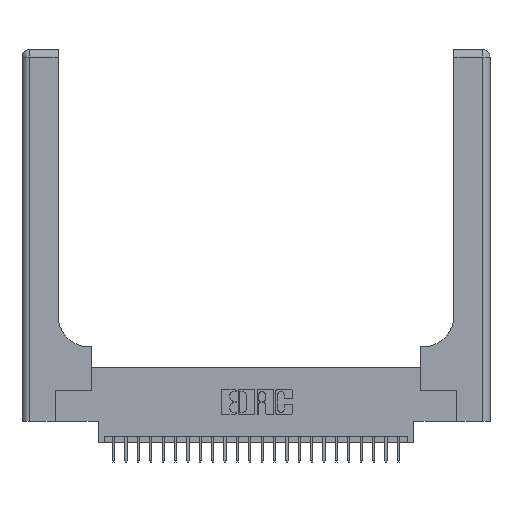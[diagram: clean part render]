
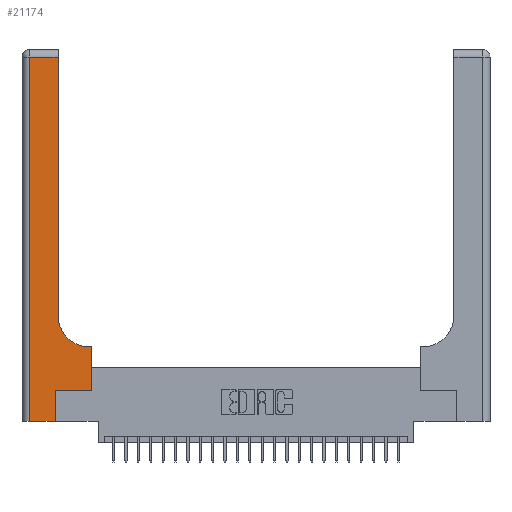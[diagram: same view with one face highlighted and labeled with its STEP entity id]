
A CAD part, top view. The second image highlights one B-rep face of the part: STEP entity #21174.
In plain terms, the highlighted planar face has unit normal (0, 0, 1).
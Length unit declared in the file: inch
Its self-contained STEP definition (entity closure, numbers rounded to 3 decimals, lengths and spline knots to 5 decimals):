
#319 = ORIENTED_EDGE ( 'NONE', *, *, #24677, .T. ) ;
#359 = EDGE_CURVE ( 'NONE', #11585, #13888, #10658, .T. ) ;
#406 = LINE ( 'NONE', #7875, #26483 ) ;
#523 = VECTOR ( 'NONE', #21432, 39.37008 ) ;
#627 = CARTESIAN_POINT ( 'NONE',  ( 0.269, 0.25, 0.37 ) ) ;
#949 = CARTESIAN_POINT ( 'NONE',  ( 0.5585, 0.25, 0.37 ) ) ;
#1217 = VERTEX_POINT ( 'NONE', #949 ) ;
#1274 = DIRECTION ( 'NONE',  ( -1., 0., 0. ) ) ;
#1945 = ORIENTED_EDGE ( 'NONE', *, *, #11618, .T. ) ;
#2642 = VERTEX_POINT ( 'NONE', #21640 ) ;
#3559 = VECTOR ( 'NONE', #11479, 39.37008 ) ;
#4810 = VECTOR ( 'NONE', #11477, 39.37008 ) ;
#5757 = VECTOR ( 'NONE', #14458, 39.37008 ) ;
#5876 = VECTOR ( 'NONE', #16796, 39.37008 ) ;
#6149 = LINE ( 'NONE', #627, #523 ) ;
#6441 = CARTESIAN_POINT ( 'NONE',  ( 0., 2.94, 0.37 ) ) ;
#6679 = CARTESIAN_POINT ( 'NONE',  ( 0.5415, 0.6, 0.37 ) ) ;
#7041 = EDGE_CURVE ( 'NONE', #7505, #15635, #25045, .T. ) ;
#7311 = AXIS2_PLACEMENT_3D ( 'NONE', #7810, #22193, #9916 ) ;
#7505 = VERTEX_POINT ( 'NONE', #21081 ) ;
#7810 = CARTESIAN_POINT ( 'NONE',  ( 0.5415, 0.85, 0.37 ) ) ;
#7875 = CARTESIAN_POINT ( 'NONE',  ( 0., 0., 0.37 ) ) ;
#8294 = AXIS2_PLACEMENT_3D ( 'NONE', #25908, #13824, #1274 ) ;
#8312 = VECTOR ( 'NONE', #22910, 39.37008 ) ;
#8372 = ORIENTED_EDGE ( 'NONE', *, *, #17217, .T. ) ;
#8820 = CARTESIAN_POINT ( 'NONE',  ( 0.2915, 2.94, 0.37 ) ) ;
#9391 = CARTESIAN_POINT ( 'NONE',  ( 0.5585, 0.25, 0.37 ) ) ;
#9601 = DIRECTION ( 'NONE',  ( 0., -1., 0. ) ) ;
#9610 = LINE ( 'NONE', #6441, #8312 ) ;
#9672 = EDGE_CURVE ( 'NONE', #2642, #1217, #6149, .T. ) ;
#9916 = DIRECTION ( 'NONE',  ( 1., 0., 0. ) ) ;
#10237 = VERTEX_POINT ( 'NONE', #8820 ) ;
#10658 = LINE ( 'NONE', #14487, #5757 ) ;
#11477 = DIRECTION ( 'NONE',  ( 0., 1., 0. ) ) ;
#11479 = DIRECTION ( 'NONE',  ( 0., 1., 0. ) ) ;
#11585 = VERTEX_POINT ( 'NONE', #22264 ) ;
#11618 = EDGE_CURVE ( 'NONE', #15635, #26148, #406, .T. ) ;
#11753 = PLANE ( 'NONE',  #8294 ) ;
#11860 = CARTESIAN_POINT ( 'NONE',  ( 0.269, 0., 0.37 ) ) ;
#12709 = ORIENTED_EDGE ( 'NONE', *, *, #359, .T. ) ;
#12786 = CIRCLE ( 'NONE', #7311, 0.25 ) ;
#13824 = DIRECTION ( 'NONE',  ( 0., 0., -1. ) ) ;
#13888 = VERTEX_POINT ( 'NONE', #6679 ) ;
#14458 = DIRECTION ( 'NONE',  ( -1., 0., 0. ) ) ;
#14487 = CARTESIAN_POINT ( 'NONE',  ( 0.2915, 0.6, 0.37 ) ) ;
#14682 = CARTESIAN_POINT ( 'NONE',  ( 0.269, 0., 0.37 ) ) ;
#15481 = EDGE_CURVE ( 'NONE', #13888, #25574, #12786, .T. ) ;
#15486 = ORIENTED_EDGE ( 'NONE', *, *, #15481, .T. ) ;
#15635 = VERTEX_POINT ( 'NONE', #22535 ) ;
#16164 = DIRECTION ( 'NONE',  ( 1., 0., 0. ) ) ;
#16796 = DIRECTION ( 'NONE',  ( 0., 1., 0. ) ) ;
#16897 = ORIENTED_EDGE ( 'NONE', *, *, #7041, .T. ) ;
#16991 = ORIENTED_EDGE ( 'NONE', *, *, #9672, .T. ) ;
#17217 = EDGE_CURVE ( 'NONE', #26148, #2642, #22329, .T. ) ;
#17624 = FACE_OUTER_BOUND ( 'NONE', #23471, .T. ) ;
#17880 = CARTESIAN_POINT ( 'NONE',  ( 0.06, 3., 0.37 ) ) ;
#19698 = ORIENTED_EDGE ( 'NONE', *, *, #22386, .T. ) ;
#19783 = VECTOR ( 'NONE', #9601, 39.37008 ) ;
#20139 = LINE ( 'NONE', #25648, #3559 ) ;
#20998 = ORIENTED_EDGE ( 'NONE', *, *, #21074, .T. ) ;
#21074 = EDGE_CURVE ( 'NONE', #25574, #10237, #20139, .T. ) ;
#21081 = CARTESIAN_POINT ( 'NONE',  ( 0.06, 2.94, 0.37 ) ) ;
#21174 = ADVANCED_FACE ( 'NONE', ( #17624 ), #11753, .F. ) ;
#21316 = LINE ( 'NONE', #9391, #4810 ) ;
#21432 = DIRECTION ( 'NONE',  ( 1., 0., 0. ) ) ;
#21640 = CARTESIAN_POINT ( 'NONE',  ( 0.269, 0.25, 0.37 ) ) ;
#21826 = CARTESIAN_POINT ( 'NONE',  ( 0.2915, 0.85, 0.37 ) ) ;
#22193 = DIRECTION ( 'NONE',  ( 0., 0., -1. ) ) ;
#22264 = CARTESIAN_POINT ( 'NONE',  ( 0.5585, 0.6, 0.37 ) ) ;
#22329 = LINE ( 'NONE', #14682, #5876 ) ;
#22386 = EDGE_CURVE ( 'NONE', #1217, #11585, #21316, .T. ) ;
#22535 = CARTESIAN_POINT ( 'NONE',  ( 0.06, 0., 0.37 ) ) ;
#22910 = DIRECTION ( 'NONE',  ( -1., 0., 0. ) ) ;
#23471 = EDGE_LOOP ( 'NONE', ( #20998, #319, #16897, #1945, #8372, #16991, #19698, #12709, #15486 ) ) ;
#24677 = EDGE_CURVE ( 'NONE', #10237, #7505, #9610, .T. ) ;
#25045 = LINE ( 'NONE', #17880, #19783 ) ;
#25574 = VERTEX_POINT ( 'NONE', #21826 ) ;
#25648 = CARTESIAN_POINT ( 'NONE',  ( 0.2915, 3., 0.37 ) ) ;
#25908 = CARTESIAN_POINT ( 'NONE',  ( 0., 3., 0.37 ) ) ;
#26148 = VERTEX_POINT ( 'NONE', #11860 ) ;
#26483 = VECTOR ( 'NONE', #16164, 39.37008 ) ;
